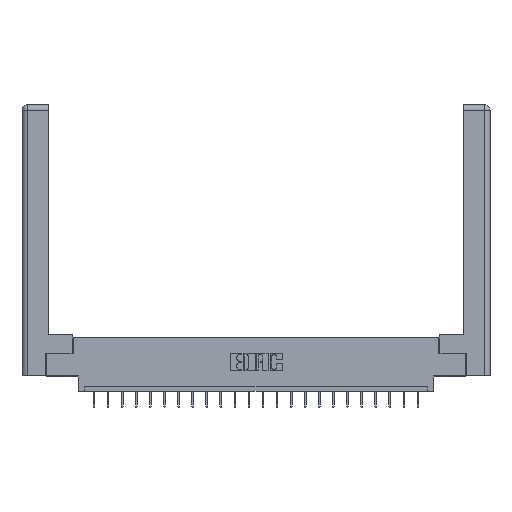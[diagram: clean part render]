
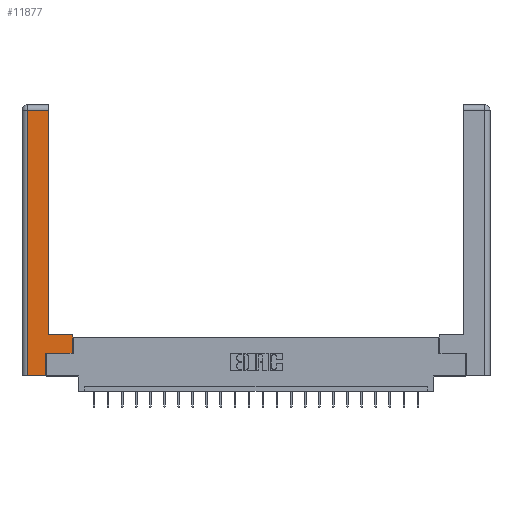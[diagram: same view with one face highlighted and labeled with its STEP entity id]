
A CAD part, top view. The second image highlights one B-rep face of the part: STEP entity #11877.
In plain terms, the highlighted planar face has unit normal (0, 0, 1).
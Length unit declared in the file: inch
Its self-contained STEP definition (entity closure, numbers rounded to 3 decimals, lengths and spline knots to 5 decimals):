
#6 = CARTESIAN_POINT ( 'NONE',  ( 0.565, 0.245, 0. ) ) ;
#426 = EDGE_CURVE ( 'NONE', #4783, #22162, #16563, .T. ) ;
#873 = CARTESIAN_POINT ( 'NONE',  ( 0.565, 0.45, 0. ) ) ;
#1240 = DIRECTION ( 'NONE',  ( -1., 0., 0. ) ) ;
#1505 = ORIENTED_EDGE ( 'NONE', *, *, #4036, .T. ) ;
#1966 = CARTESIAN_POINT ( 'NONE',  ( 0.565, 0.45, 0. ) ) ;
#2967 = VERTEX_POINT ( 'NONE', #20489 ) ;
#3080 = CARTESIAN_POINT ( 'NONE',  ( 0., 0., 0. ) ) ;
#3147 = PLANE ( 'NONE',  #12760 ) ;
#3178 = ORIENTED_EDGE ( 'NONE', *, *, #22366, .T. ) ;
#3463 = LINE ( 'NONE', #18181, #13774 ) ;
#3474 = DIRECTION ( 'NONE',  ( -1., 0., 0. ) ) ;
#4036 = EDGE_CURVE ( 'NONE', #10280, #9080, #18386, .T. ) ;
#4215 = EDGE_CURVE ( 'NONE', #8546, #22004, #6351, .T. ) ;
#4254 = DIRECTION ( 'NONE',  ( 0., -1., 0. ) ) ;
#4319 = VERTEX_POINT ( 'NONE', #18235 ) ;
#4783 = VERTEX_POINT ( 'NONE', #10860 ) ;
#5011 = EDGE_CURVE ( 'NONE', #4319, #4783, #8543, .T. ) ;
#5114 = VECTOR ( 'NONE', #6081, 39.37008 ) ;
#5677 = VECTOR ( 'NONE', #4254, 39.37008 ) ;
#6081 = DIRECTION ( 'NONE',  ( -1., 0., 0. ) ) ;
#6351 = LINE ( 'NONE', #1966, #12790 ) ;
#6862 = ORIENTED_EDGE ( 'NONE', *, *, #18789, .T. ) ;
#7156 = DIRECTION ( 'NONE',  ( 0., 1., 0. ) ) ;
#7566 = DIRECTION ( 'NONE',  ( 1., 0., 0. ) ) ;
#7893 = CARTESIAN_POINT ( 'NONE',  ( 0.295, 3., 0. ) ) ;
#8543 = LINE ( 'NONE', #7893, #19713 ) ;
#8546 = VERTEX_POINT ( 'NONE', #6 ) ;
#9080 = VERTEX_POINT ( 'NONE', #11933 ) ;
#9439 = CARTESIAN_POINT ( 'NONE',  ( 0.265, 0., 0. ) ) ;
#9548 = EDGE_CURVE ( 'NONE', #2967, #10280, #19395, .T. ) ;
#10239 = ORIENTED_EDGE ( 'NONE', *, *, #9548, .T. ) ;
#10280 = VERTEX_POINT ( 'NONE', #20593 ) ;
#10860 = CARTESIAN_POINT ( 'NONE',  ( 0.295, 2.94, 0. ) ) ;
#11877 = ADVANCED_FACE ( 'NONE', ( #21638 ), #3147, .F. ) ;
#11933 = CARTESIAN_POINT ( 'NONE',  ( 0.265, 0.245, 0. ) ) ;
#12194 = ORIENTED_EDGE ( 'NONE', *, *, #5011, .T. ) ;
#12369 = LINE ( 'NONE', #20706, #5677 ) ;
#12760 = AXIS2_PLACEMENT_3D ( 'NONE', #3080, #15425, #1240 ) ;
#12790 = VECTOR ( 'NONE', #7156, 39.37008 ) ;
#13262 = ORIENTED_EDGE ( 'NONE', *, *, #426, .T. ) ;
#13757 = DIRECTION ( 'NONE',  ( 0., 1., 0. ) ) ;
#13774 = VECTOR ( 'NONE', #7566, 39.37008 ) ;
#14488 = VECTOR ( 'NONE', #19268, 39.37008 ) ;
#14675 = CARTESIAN_POINT ( 'NONE',  ( 0.0615, 2.94, 0. ) ) ;
#14825 = VECTOR ( 'NONE', #3474, 39.37008 ) ;
#15425 = DIRECTION ( 'NONE',  ( 0., 0., -1. ) ) ;
#16416 = EDGE_CURVE ( 'NONE', #22162, #2967, #12369, .T. ) ;
#16563 = LINE ( 'NONE', #14675, #5114 ) ;
#16664 = DIRECTION ( 'NONE',  ( 1., 0., 0. ) ) ;
#17242 = CARTESIAN_POINT ( 'NONE',  ( 0.0615, 2.94, 0. ) ) ;
#17544 = ORIENTED_EDGE ( 'NONE', *, *, #16416, .T. ) ;
#17722 = ORIENTED_EDGE ( 'NONE', *, *, #4215, .T. ) ;
#17847 = LINE ( 'NONE', #21094, #14825 ) ;
#18181 = CARTESIAN_POINT ( 'NONE',  ( 0.565, 0.245, 0. ) ) ;
#18235 = CARTESIAN_POINT ( 'NONE',  ( 0.295, 0.45, 0. ) ) ;
#18386 = LINE ( 'NONE', #22503, #14488 ) ;
#18556 = VECTOR ( 'NONE', #16664, 39.37008 ) ;
#18789 = EDGE_CURVE ( 'NONE', #22004, #4319, #17847, .T. ) ;
#19268 = DIRECTION ( 'NONE',  ( 0., 1., 0. ) ) ;
#19395 = LINE ( 'NONE', #9439, #18556 ) ;
#19713 = VECTOR ( 'NONE', #13757, 39.37008 ) ;
#20489 = CARTESIAN_POINT ( 'NONE',  ( 0.0615, 0., 0. ) ) ;
#20593 = CARTESIAN_POINT ( 'NONE',  ( 0.265, 0., 0. ) ) ;
#20706 = CARTESIAN_POINT ( 'NONE',  ( 0.0615, 0., 0. ) ) ;
#21094 = CARTESIAN_POINT ( 'NONE',  ( 0.295, 0.45, 0. ) ) ;
#21638 = FACE_OUTER_BOUND ( 'NONE', #22703, .T. ) ;
#22004 = VERTEX_POINT ( 'NONE', #873 ) ;
#22162 = VERTEX_POINT ( 'NONE', #17242 ) ;
#22366 = EDGE_CURVE ( 'NONE', #9080, #8546, #3463, .T. ) ;
#22503 = CARTESIAN_POINT ( 'NONE',  ( 0.265, 0.245, 0. ) ) ;
#22703 = EDGE_LOOP ( 'NONE', ( #12194, #13262, #17544, #10239, #1505, #3178, #17722, #6862 ) ) ;
